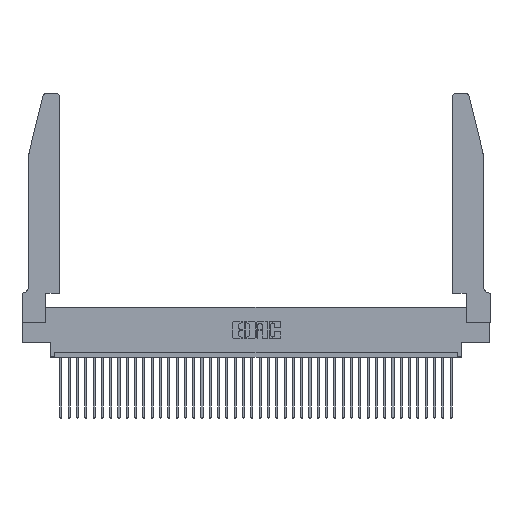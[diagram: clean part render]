
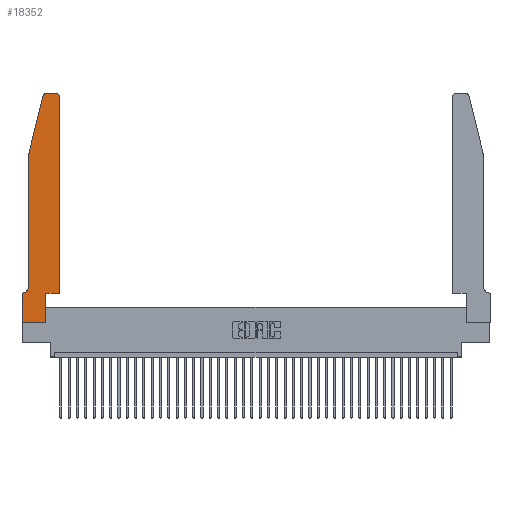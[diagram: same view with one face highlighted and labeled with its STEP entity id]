
A CAD part, top view. The second image highlights one B-rep face of the part: STEP entity #18352.
In plain terms, the highlighted planar face has unit normal (0, 0, 1).
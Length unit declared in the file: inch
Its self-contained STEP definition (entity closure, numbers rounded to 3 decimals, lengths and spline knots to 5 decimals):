
#882 = CARTESIAN_POINT ( 'NONE',  ( 0.4505, 0.35, 0.37 ) ) ;
#1995 = EDGE_CURVE ( 'NONE', #20659, #4190, #3210, .T. ) ;
#2708 = VERTEX_POINT ( 'NONE', #14218 ) ;
#2726 = VECTOR ( 'NONE', #6240, 39.37008 ) ;
#2883 = VECTOR ( 'NONE', #3267, 39.37008 ) ;
#3210 = LINE ( 'NONE', #13360, #18719 ) ;
#3267 = DIRECTION ( 'NONE',  ( -1., 0., 0. ) ) ;
#3324 = EDGE_CURVE ( 'NONE', #3937, #20659, #4544, .T. ) ;
#3937 = VERTEX_POINT ( 'NONE', #4609 ) ;
#4035 = ORIENTED_EDGE ( 'NONE', *, *, #1995, .T. ) ;
#4049 = DIRECTION ( 'NONE',  ( -0.239, -0.971, 0. ) ) ;
#4069 = ORIENTED_EDGE ( 'NONE', *, *, #16125, .T. ) ;
#4190 = VERTEX_POINT ( 'NONE', #21423 ) ;
#4291 = EDGE_CURVE ( 'NONE', #4190, #2708, #36118, .T. ) ;
#4315 = LINE ( 'NONE', #9730, #2883 ) ;
#4519 = ORIENTED_EDGE ( 'NONE', *, *, #16448, .T. ) ;
#4544 = LINE ( 'NONE', #20305, #15649 ) ;
#4609 = CARTESIAN_POINT ( 'NONE',  ( 0.2865, 0., 0.37 ) ) ;
#4881 = ORIENTED_EDGE ( 'NONE', *, *, #14357, .T. ) ;
#5128 = VERTEX_POINT ( 'NONE', #32574 ) ;
#5293 = ORIENTED_EDGE ( 'NONE', *, *, #26991, .T. ) ;
#5457 = VERTEX_POINT ( 'NONE', #31582 ) ;
#5709 = AXIS2_PLACEMENT_3D ( 'NONE', #28275, #37303, #9664 ) ;
#6240 = DIRECTION ( 'NONE',  ( 0., -1., 0. ) ) ;
#6780 = ORIENTED_EDGE ( 'NONE', *, *, #4291, .T. ) ;
#7182 = CARTESIAN_POINT ( 'NONE',  ( 0.25487, 2.72718, 0.37 ) ) ;
#8596 = CARTESIAN_POINT ( 'NONE',  ( 0.284, 2.75, 0.37 ) ) ;
#9180 = CIRCLE ( 'NONE', #5709, 0.07 ) ;
#9664 = DIRECTION ( 'NONE',  ( -1., 0., 0. ) ) ;
#9730 = CARTESIAN_POINT ( 'NONE',  ( 0.0755, 0.35, 0.37 ) ) ;
#9877 = DIRECTION ( 'NONE',  ( 1., 0., 0. ) ) ;
#10510 = EDGE_CURVE ( 'NONE', #38332, #5457, #18716, .T. ) ;
#10953 = CARTESIAN_POINT ( 'NONE',  ( 0.0755, 2., 0.37 ) ) ;
#11113 = VERTEX_POINT ( 'NONE', #27818 ) ;
#11199 = CIRCLE ( 'NONE', #32117, 0.03 ) ;
#11360 = LINE ( 'NONE', #39264, #20557 ) ;
#12653 = PLANE ( 'NONE',  #36236 ) ;
#13213 = DIRECTION ( 'NONE',  ( 0., 0., 1. ) ) ;
#13360 = CARTESIAN_POINT ( 'NONE',  ( 0.4505, 0.35, 0.37 ) ) ;
#13627 = EDGE_CURVE ( 'NONE', #14641, #3937, #11360, .T. ) ;
#13704 = VERTEX_POINT ( 'NONE', #7182 ) ;
#14218 = CARTESIAN_POINT ( 'NONE',  ( 0.4505, 2.72, 0.37 ) ) ;
#14357 = EDGE_CURVE ( 'NONE', #27177, #15680, #15148, .T. ) ;
#14432 = DIRECTION ( 'NONE',  ( 1., 0., 0. ) ) ;
#14641 = VERTEX_POINT ( 'NONE', #16220 ) ;
#15148 = LINE ( 'NONE', #28814, #20020 ) ;
#15514 = EDGE_CURVE ( 'NONE', #15680, #13704, #11199, .T. ) ;
#15649 = VECTOR ( 'NONE', #32870, 39.37008 ) ;
#15680 = VERTEX_POINT ( 'NONE', #8596 ) ;
#16125 = EDGE_CURVE ( 'NONE', #5128, #14641, #33502, .T. ) ;
#16220 = CARTESIAN_POINT ( 'NONE',  ( 0., 0., 0.37 ) ) ;
#16448 = EDGE_CURVE ( 'NONE', #13704, #38332, #36429, .T. ) ;
#17047 = CARTESIAN_POINT ( 'NONE',  ( 0., 0.35, 0.37 ) ) ;
#17219 = CARTESIAN_POINT ( 'NONE',  ( 0.284, 2.72, 0.37 ) ) ;
#18352 = ADVANCED_FACE ( 'NONE', ( #37861 ), #12653, .T. ) ;
#18376 = DIRECTION ( 'NONE',  ( 0., -1., 0. ) ) ;
#18716 = LINE ( 'NONE', #24777, #2726 ) ;
#18719 = VECTOR ( 'NONE', #9877, 39.37008 ) ;
#20020 = VECTOR ( 'NONE', #31956, 39.37008 ) ;
#20216 = CIRCLE ( 'NONE', #38260, 0.03 ) ;
#20305 = CARTESIAN_POINT ( 'NONE',  ( 0.2865, 0.35, 0.37 ) ) ;
#20557 = VECTOR ( 'NONE', #29997, 39.37008 ) ;
#20659 = VERTEX_POINT ( 'NONE', #24087 ) ;
#21423 = CARTESIAN_POINT ( 'NONE',  ( 0.4505, 0.35, 0.37 ) ) ;
#21846 = CARTESIAN_POINT ( 'NONE',  ( 0., 0., 0.37 ) ) ;
#23752 = ORIENTED_EDGE ( 'NONE', *, *, #10510, .T. ) ;
#24087 = CARTESIAN_POINT ( 'NONE',  ( 0.2865, 0.35, 0.37 ) ) ;
#24777 = CARTESIAN_POINT ( 'NONE',  ( 0.0755, 2., 0.37 ) ) ;
#25220 = EDGE_LOOP ( 'NONE', ( #4881, #27422, #4519, #23752, #31277, #39220, #4069, #31193, #27145, #4035, #6780, #5293 ) ) ;
#25779 = DIRECTION ( 'NONE',  ( 0., 1., 0. ) ) ;
#25847 = VECTOR ( 'NONE', #25779, 39.37008 ) ;
#25902 = EDGE_CURVE ( 'NONE', #5457, #11113, #9180, .T. ) ;
#26191 = CARTESIAN_POINT ( 'NONE',  ( 0.4205, 2.75, 0.37 ) ) ;
#26991 = EDGE_CURVE ( 'NONE', #2708, #27177, #20216, .T. ) ;
#27145 = ORIENTED_EDGE ( 'NONE', *, *, #3324, .T. ) ;
#27149 = VECTOR ( 'NONE', #4049, 39.37008 ) ;
#27177 = VERTEX_POINT ( 'NONE', #26191 ) ;
#27422 = ORIENTED_EDGE ( 'NONE', *, *, #15514, .T. ) ;
#27818 = CARTESIAN_POINT ( 'NONE',  ( 0.0055, 0.35, 0.37 ) ) ;
#28275 = CARTESIAN_POINT ( 'NONE',  ( 0.0055, 0.42, 0.37 ) ) ;
#28814 = CARTESIAN_POINT ( 'NONE',  ( 0.2605, 2.75, 0.37 ) ) ;
#29997 = DIRECTION ( 'NONE',  ( 1., 0., 0. ) ) ;
#30179 = CARTESIAN_POINT ( 'NONE',  ( 0.0755, 2., 0.37 ) ) ;
#31193 = ORIENTED_EDGE ( 'NONE', *, *, #13627, .T. ) ;
#31277 = ORIENTED_EDGE ( 'NONE', *, *, #25902, .T. ) ;
#31582 = CARTESIAN_POINT ( 'NONE',  ( 0.0755, 0.42, 0.37 ) ) ;
#31846 = EDGE_CURVE ( 'NONE', #11113, #5128, #4315, .T. ) ;
#31896 = CARTESIAN_POINT ( 'NONE',  ( 0.4205, 2.72, 0.37 ) ) ;
#31956 = DIRECTION ( 'NONE',  ( -1., 0., 0. ) ) ;
#32117 = AXIS2_PLACEMENT_3D ( 'NONE', #17219, #33105, #14432 ) ;
#32574 = CARTESIAN_POINT ( 'NONE',  ( 0., 0.35, 0.37 ) ) ;
#32704 = DIRECTION ( 'NONE',  ( 0., 0., 1. ) ) ;
#32840 = DIRECTION ( 'NONE',  ( 1., 0., 0. ) ) ;
#32870 = DIRECTION ( 'NONE',  ( 0., 1., 0. ) ) ;
#33105 = DIRECTION ( 'NONE',  ( 0., 0., 1. ) ) ;
#33502 = LINE ( 'NONE', #21846, #39386 ) ;
#36118 = LINE ( 'NONE', #882, #25847 ) ;
#36236 = AXIS2_PLACEMENT_3D ( 'NONE', #17047, #32704, #32840 ) ;
#36429 = LINE ( 'NONE', #30179, #27149 ) ;
#37303 = DIRECTION ( 'NONE',  ( 0., 0., -1. ) ) ;
#37861 = FACE_OUTER_BOUND ( 'NONE', #25220, .T. ) ;
#38155 = DIRECTION ( 'NONE',  ( 1., 0., 0. ) ) ;
#38260 = AXIS2_PLACEMENT_3D ( 'NONE', #31896, #13213, #38155 ) ;
#38332 = VERTEX_POINT ( 'NONE', #10953 ) ;
#39220 = ORIENTED_EDGE ( 'NONE', *, *, #31846, .T. ) ;
#39264 = CARTESIAN_POINT ( 'NONE',  ( 0., 0., 0.37 ) ) ;
#39386 = VECTOR ( 'NONE', #18376, 39.37008 ) ;
